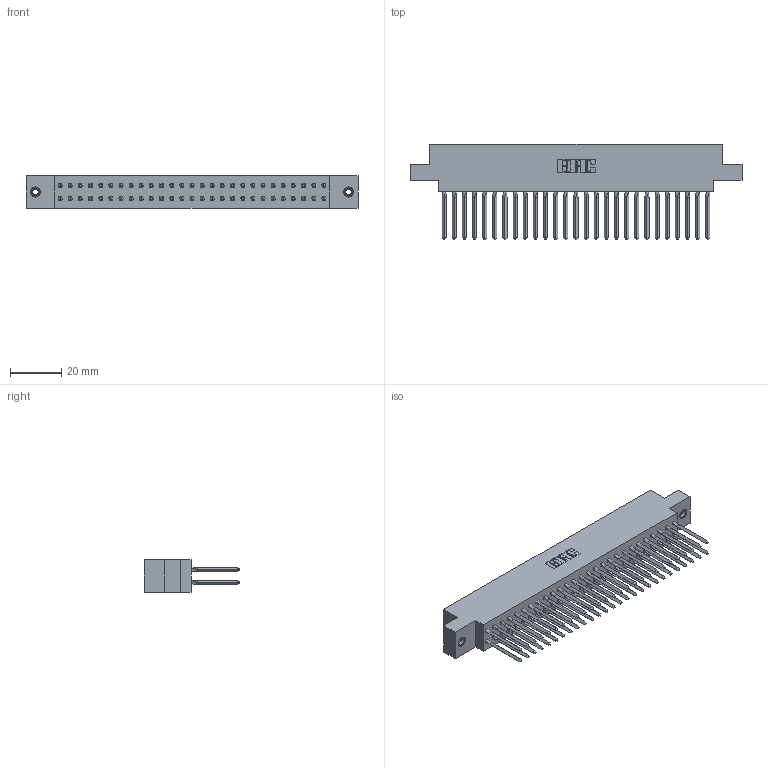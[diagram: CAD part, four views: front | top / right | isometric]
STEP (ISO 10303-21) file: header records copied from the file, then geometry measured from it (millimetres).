
FILE_DESCRIPTION (( 'STEP AP203' ), '1' );
FILE_NAME ('317-054-542-808.STEP', '2020-02-28T03:59:19', ( '' ), ( '' ), 'SwSTEP 2.0', 'SolidWorks 2016', '' );
FILE_SCHEMA (( 'CONFIG_CONTROL_DESIGN' ));
Length unit declared in the file: inch
Products named in the file (4): 345-250-001_345-250-003-102; 317 Part_.156 Dia - TI; 317-290-003_542; 317-054-542-808
Assembly tree (57 placements, depth 2):
  317-054-542-808
    317 Part_.156 Dia - TI
    317-290-003_542  x54
    345-250-001_345-250-003-102  x2
Bounding box: 129.69 x 37.34 x 12.7 mm (x, y, z)
Volume: 20756.1 mm3; surface area: 28404.5 mm2
Topology: 57 solids, 57 shells, 3240 faces, 9051 edges, 5774 vertices
Faces by surface type: plane 2574, cylinder 434, bspline 216, cone 12, torus 4
Entity records: 41324 total; most frequent: CARTESIAN_POINT 7428, ORIENTED_EDGE 7084, DIRECTION 6024, EDGE_CURVE 3542, VECTOR 3352, LINE 3352, VERTEX_POINT 2352, AXIS2_PLACEMENT_3D 1336
